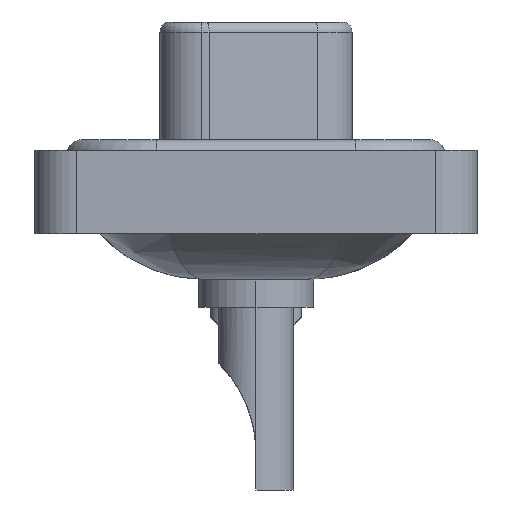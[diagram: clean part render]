
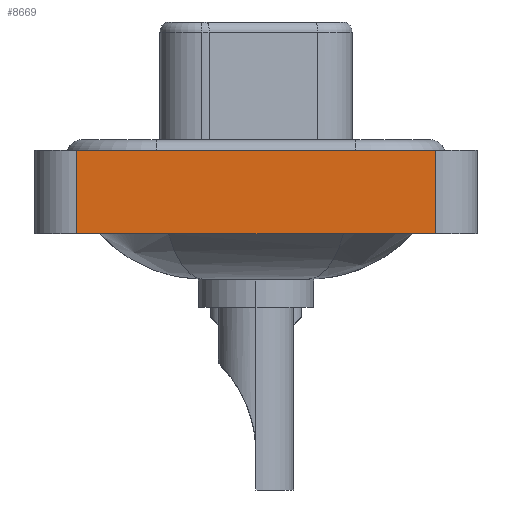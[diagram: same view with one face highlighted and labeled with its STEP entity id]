
A CAD part, left-side view. The second image highlights one B-rep face of the part: STEP entity #8669.
In plain terms, the highlighted planar face has unit normal (-1, 0, 0).
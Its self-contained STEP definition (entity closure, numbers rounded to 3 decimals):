
#601 = VECTOR ( 'NONE', #12898, 1000. ) ;
#603 = EDGE_LOOP ( 'NONE', ( #5021, #17212, #12925, #18098 ) ) ;
#950 = CARTESIAN_POINT ( 'NONE',  ( -7.3, -8.55, -3.6 ) ) ;
#991 = LINE ( 'NONE', #8466, #15370 ) ;
#1266 = CARTESIAN_POINT ( 'NONE',  ( -7.3, 8.55, -3.6 ) ) ;
#2106 = EDGE_CURVE ( 'NONE', #12512, #11301, #5327, .T. ) ;
#2354 = VERTEX_POINT ( 'NONE', #19297 ) ;
#3851 = DIRECTION ( 'NONE',  ( 0., 0., 1. ) ) ;
#3854 = LINE ( 'NONE', #5338, #601 ) ;
#3884 = EDGE_CURVE ( 'NONE', #18204, #12512, #991, .T. ) ;
#5021 = ORIENTED_EDGE ( 'NONE', *, *, #2106, .T. ) ;
#5327 = LINE ( 'NONE', #950, #13927 ) ;
#5338 = CARTESIAN_POINT ( 'NONE',  ( -7.3, -8.55, 0.4 ) ) ;
#5424 = PLANE ( 'NONE',  #5924 ) ;
#5924 = AXIS2_PLACEMENT_3D ( 'NONE', #9830, #15680, #3851 ) ;
#6292 = VECTOR ( 'NONE', #7339, 1000. ) ;
#6882 = DIRECTION ( 'NONE',  ( 0., -1., 0. ) ) ;
#7018 = DIRECTION ( 'NONE',  ( 0., 0., 1. ) ) ;
#7339 = DIRECTION ( 'NONE',  ( 0., 0., 1. ) ) ;
#8133 = FACE_OUTER_BOUND ( 'NONE', #603, .T. ) ;
#8466 = CARTESIAN_POINT ( 'NONE',  ( -7.3, -8.55, -3.6 ) ) ;
#8669 = ADVANCED_FACE ( 'NONE', ( #8133 ), #5424, .T. ) ;
#9507 = EDGE_CURVE ( 'NONE', #18204, #2354, #17971, .T. ) ;
#9680 = EDGE_CURVE ( 'NONE', #2354, #11301, #3854, .T. ) ;
#9830 = CARTESIAN_POINT ( 'NONE',  ( -7.3, -8.55, -3.6 ) ) ;
#10109 = CARTESIAN_POINT ( 'NONE',  ( -7.3, 8.55, -3.6 ) ) ;
#11301 = VERTEX_POINT ( 'NONE', #16551 ) ;
#12512 = VERTEX_POINT ( 'NONE', #17655 ) ;
#12898 = DIRECTION ( 'NONE',  ( 0., -1., 0. ) ) ;
#12925 = ORIENTED_EDGE ( 'NONE', *, *, #9507, .F. ) ;
#13927 = VECTOR ( 'NONE', #7018, 1000. ) ;
#15370 = VECTOR ( 'NONE', #6882, 1000. ) ;
#15680 = DIRECTION ( 'NONE',  ( -1., 0., 0. ) ) ;
#16551 = CARTESIAN_POINT ( 'NONE',  ( -7.3, -8.55, 0.4 ) ) ;
#17212 = ORIENTED_EDGE ( 'NONE', *, *, #9680, .F. ) ;
#17655 = CARTESIAN_POINT ( 'NONE',  ( -7.3, -8.55, -3.6 ) ) ;
#17971 = LINE ( 'NONE', #1266, #6292 ) ;
#18098 = ORIENTED_EDGE ( 'NONE', *, *, #3884, .T. ) ;
#18204 = VERTEX_POINT ( 'NONE', #10109 ) ;
#19297 = CARTESIAN_POINT ( 'NONE',  ( -7.3, 8.55, 0.4 ) ) ;
